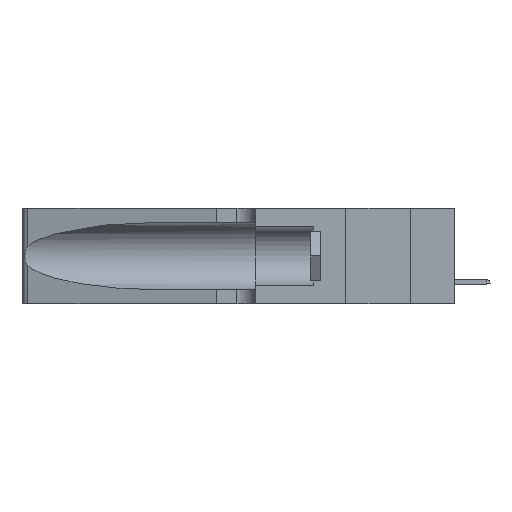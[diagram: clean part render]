
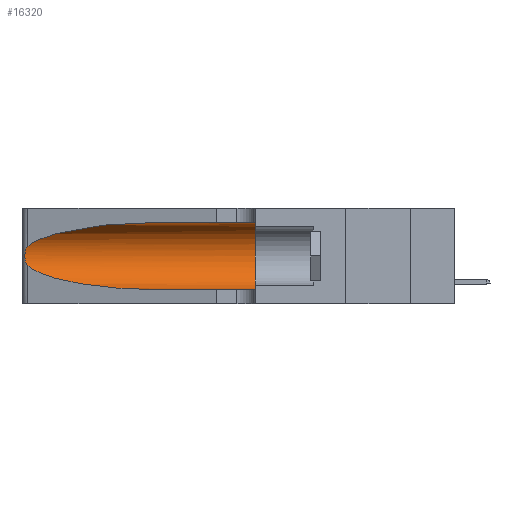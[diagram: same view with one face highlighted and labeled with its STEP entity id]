
A CAD part, left-side view. The second image highlights one B-rep face of the part: STEP entity #16320.
In plain terms, the highlighted cylindrical face has radius 3.308 mm (diameter 6.617 mm), a partial arc.
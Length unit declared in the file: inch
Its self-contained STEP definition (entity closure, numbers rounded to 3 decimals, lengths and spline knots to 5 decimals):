
#552 = CARTESIAN_POINT ( 'NONE',  ( 0.26018, 1.23835, 0.19895 ) ) ;
#900 = ORIENTED_EDGE ( 'NONE', *, *, #13983, .F. ) ;
#1259 = EDGE_CURVE ( 'NONE', #31324, #12467, #4268, .T. ) ;
#2151 = CARTESIAN_POINT ( 'NONE',  ( 0.1305, 0.35, 0.05475 ) ) ;
#3745 = VERTEX_POINT ( 'NONE', #8833 ) ;
#4108 = AXIS2_PLACEMENT_3D ( 'NONE', #35162, #18401, #31197 ) ;
#4268 =( BOUNDED_CURVE ( )  B_SPLINE_CURVE ( 3, ( #31203, #11706, #37278, #21977 ),
 .UNSPECIFIED., .F., .T. ) 
 B_SPLINE_CURVE_WITH_KNOTS ( ( 4, 4 ),
 ( 3.44316, 4.71239 ),
 .UNSPECIFIED. ) 
 CURVE ( )  GEOMETRIC_REPRESENTATION_ITEM ( )  RATIONAL_B_SPLINE_CURVE ( ( 1., 0.87, 0.87, 1. ) ) 
 REPRESENTATION_ITEM ( '' )  );
#6241 = CARTESIAN_POINT ( 'NONE',  ( 0.25787, 1.23484, 0.2124 ) ) ;
#6842 = CARTESIAN_POINT ( 'NONE',  ( 0.26075, 1.23896, 0.19203 ) ) ;
#7103 = DIRECTION ( 'NONE',  ( 0., 1., 0. ) ) ;
#8298 = VERTEX_POINT ( 'NONE', #10582 ) ;
#8833 = CARTESIAN_POINT ( 'NONE',  ( 0.1305, 0.35, 0.31525 ) ) ;
#9342 = DIRECTION ( 'NONE',  ( 0., -1., 0. ) ) ;
#9782 = CARTESIAN_POINT ( 'NONE',  ( 0.26075, 1.23896, 0.178 ) ) ;
#9985 = CARTESIAN_POINT ( 'NONE',  ( 0.25789, 1.23486, 0.15765 ) ) ;
#10582 = CARTESIAN_POINT ( 'NONE',  ( 0.1305, 0.72297, 0.31525 ) ) ;
#11706 = CARTESIAN_POINT ( 'NONE',  ( 0.2373, 1.15595, 0.08982 ) ) ;
#11736 = VERTEX_POINT ( 'NONE', #2151 ) ;
#12467 = VERTEX_POINT ( 'NONE', #29885 ) ;
#12471 = EDGE_CURVE ( 'NONE', #12467, #11736, #36176, .T. ) ;
#12859 = CARTESIAN_POINT ( 'NONE',  ( 0.18966, 0.96281, 0.31525 ) ) ;
#13340 = CARTESIAN_POINT ( 'NONE',  ( 0.25856, 1.23593, 0.16098 ) ) ;
#13660 = CARTESIAN_POINT ( 'NONE',  ( 0.25487, 1.22718, 0.22369 ) ) ;
#13983 = EDGE_CURVE ( 'NONE', #8298, #3745, #18358, .T. ) ;
#14384 = ORIENTED_EDGE ( 'NONE', *, *, #12471, .T. ) ;
#14522 = EDGE_CURVE ( 'NONE', #8298, #34658, #34268, .T. ) ;
#15677 = CYLINDRICAL_SURFACE ( 'NONE', #4108, 0.13025 ) ;
#16035 = VECTOR ( 'NONE', #9342, 39.37008 ) ;
#16075 = CARTESIAN_POINT ( 'NONE',  ( 0.25854, 1.2359, 0.20912 ) ) ;
#16118 = ORIENTED_EDGE ( 'NONE', *, *, #40350, .F. ) ;
#16320 = ADVANCED_FACE ( 'NONE', ( #39972 ), #15677, .F. ) ;
#16475 = CARTESIAN_POINT ( 'NONE',  ( 0.25487, 1.22718, 0.22369 ) ) ;
#18249 = ORIENTED_EDGE ( 'NONE', *, *, #38121, .T. ) ;
#18358 = LINE ( 'NONE', #18983, #16035 ) ;
#18401 = DIRECTION ( 'NONE',  ( 0., -1., 0. ) ) ;
#18983 = CARTESIAN_POINT ( 'NONE',  ( 0.1305, 1.61858, 0.31525 ) ) ;
#19068 = CARTESIAN_POINT ( 'NONE',  ( 0.25487, 1.22718, 0.22369 ) ) ;
#19219 = CARTESIAN_POINT ( 'NONE',  ( 0.25639, 1.23186, 0.15144 ) ) ;
#19516 = ORIENTED_EDGE ( 'NONE', *, *, #14522, .T. ) ;
#20038 = VECTOR ( 'NONE', #26509, 39.37008 ) ;
#20413 = B_SPLINE_CURVE_WITH_KNOTS ( 'NONE', 3,
 ( #16475, #38493, #25677, #6241, #16075, #552, #6842, #9782, #33177, #13340, #9985, #19219, #26090, #30033 ),
 .UNSPECIFIED., .F., .F.,
 ( 4, 2, 2, 2, 2, 2, 4 ),
 ( 0., 0.00027, 0.00053, 0.00107, 0.0016, 0.00187, 0.00214 ),
 .UNSPECIFIED. ) ;
#21977 = CARTESIAN_POINT ( 'NONE',  ( 0.1305, 0.72297, 0.05475 ) ) ;
#22386 = ORIENTED_EDGE ( 'NONE', *, *, #1259, .T. ) ;
#22972 = CARTESIAN_POINT ( 'NONE',  ( 0.1305, 1.61858, 0.05475 ) ) ;
#25677 = CARTESIAN_POINT ( 'NONE',  ( 0.25639, 1.23184, 0.21858 ) ) ;
#25738 = CARTESIAN_POINT ( 'NONE',  ( 0.1305, 0.35, 0.185 ) ) ;
#26090 = CARTESIAN_POINT ( 'NONE',  ( 0.25555, 1.22993, 0.14849 ) ) ;
#26509 = DIRECTION ( 'NONE',  ( 0., -1., 0. ) ) ;
#28452 = CARTESIAN_POINT ( 'NONE',  ( 0.25487, 1.22718, 0.14631 ) ) ;
#29581 = CARTESIAN_POINT ( 'NONE',  ( 0.1305, 0.72297, 0.31525 ) ) ;
#29885 = CARTESIAN_POINT ( 'NONE',  ( 0.1305, 0.72297, 0.05475 ) ) ;
#30033 = CARTESIAN_POINT ( 'NONE',  ( 0.25487, 1.22718, 0.14631 ) ) ;
#31197 = DIRECTION ( 'NONE',  ( 0., 0., -1. ) ) ;
#31203 = CARTESIAN_POINT ( 'NONE',  ( 0.25487, 1.22718, 0.14631 ) ) ;
#31324 = VERTEX_POINT ( 'NONE', #28452 ) ;
#32134 = CARTESIAN_POINT ( 'NONE',  ( 0.2373, 1.15595, 0.28018 ) ) ;
#32156 = EDGE_LOOP ( 'NONE', ( #19516, #18249, #22386, #14384, #16118, #900 ) ) ;
#33177 = CARTESIAN_POINT ( 'NONE',  ( 0.26017, 1.23833, 0.17102 ) ) ;
#34268 =( BOUNDED_CURVE ( )  B_SPLINE_CURVE ( 3, ( #29581, #12859, #32134, #13660 ),
 .UNSPECIFIED., .F., .T. ) 
 B_SPLINE_CURVE_WITH_KNOTS ( ( 4, 4 ),
 ( 1.5708, 2.84003 ),
 .UNSPECIFIED. ) 
 CURVE ( )  GEOMETRIC_REPRESENTATION_ITEM ( )  RATIONAL_B_SPLINE_CURVE ( ( 1., 0.87, 0.87, 1. ) ) 
 REPRESENTATION_ITEM ( '' )  );
#34658 = VERTEX_POINT ( 'NONE', #19068 ) ;
#35162 = CARTESIAN_POINT ( 'NONE',  ( 0.1305, 1.61858, 0.185 ) ) ;
#35609 = DIRECTION ( 'NONE',  ( 0., 0., 1. ) ) ;
#36176 = LINE ( 'NONE', #22972, #20038 ) ;
#37278 = CARTESIAN_POINT ( 'NONE',  ( 0.18966, 0.96281, 0.05475 ) ) ;
#37778 = CIRCLE ( 'NONE', #39750, 0.13025 ) ;
#38121 = EDGE_CURVE ( 'NONE', #34658, #31324, #20413, .T. ) ;
#38493 = CARTESIAN_POINT ( 'NONE',  ( 0.25555, 1.22994, 0.2215 ) ) ;
#39750 = AXIS2_PLACEMENT_3D ( 'NONE', #25738, #7103, #35609 ) ;
#39972 = FACE_OUTER_BOUND ( 'NONE', #32156, .T. ) ;
#40350 = EDGE_CURVE ( 'NONE', #3745, #11736, #37778, .T. ) ;
